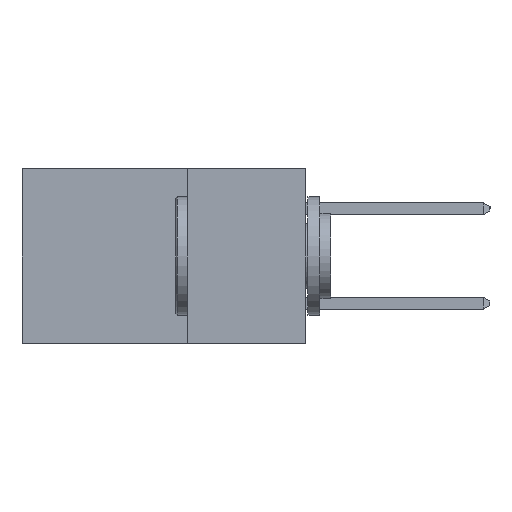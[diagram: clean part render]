
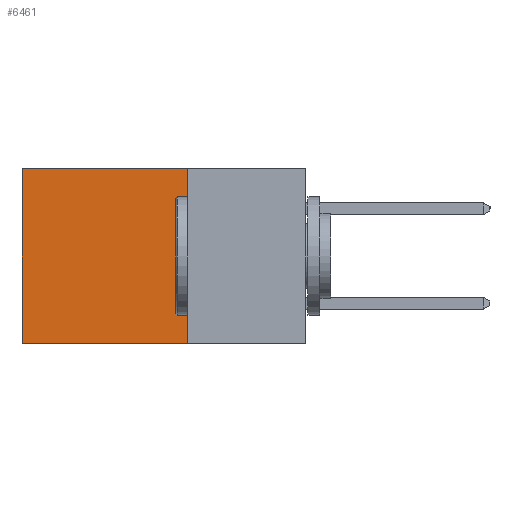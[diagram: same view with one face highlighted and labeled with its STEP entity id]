
A CAD part, left-side view. The second image highlights one B-rep face of the part: STEP entity #6461.
In plain terms, the highlighted planar face has unit normal (-1, 0, 0).
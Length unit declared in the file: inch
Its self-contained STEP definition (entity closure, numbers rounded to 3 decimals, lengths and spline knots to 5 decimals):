
#2274 = VECTOR ( 'NONE', #8849, 39.37008 ) ;
#3377 = EDGE_CURVE ( 'NONE', #10340, #13075, #22124, .T. ) ;
#3886 = VERTEX_POINT ( 'NONE', #10291 ) ;
#3919 = CARTESIAN_POINT ( 'NONE',  ( 0.2615, 0.25, 0. ) ) ;
#4617 = CARTESIAN_POINT ( 'NONE',  ( 0.2615, 0.25, -0.37 ) ) ;
#4715 = LINE ( 'NONE', #7134, #2274 ) ;
#5074 = CARTESIAN_POINT ( 'NONE',  ( 0.2615, 0.25, -0.37 ) ) ;
#6045 = CARTESIAN_POINT ( 'NONE',  ( 0.2615, 0.25, -0.37 ) ) ;
#6405 = ORIENTED_EDGE ( 'NONE', *, *, #15888, .F. ) ;
#6461 = ADVANCED_FACE ( 'NONE', ( #10420 ), #21023, .F. ) ;
#7134 = CARTESIAN_POINT ( 'NONE',  ( 0.2615, 0.6, -0.37 ) ) ;
#8092 = VERTEX_POINT ( 'NONE', #20190 ) ;
#8849 = DIRECTION ( 'NONE',  ( 0., 0., -1. ) ) ;
#9092 = DIRECTION ( 'NONE',  ( 0., 1., 0. ) ) ;
#9520 = VECTOR ( 'NONE', #9092, 39.37008 ) ;
#9632 = EDGE_CURVE ( 'NONE', #10340, #8092, #20566, .T. ) ;
#10031 = DIRECTION ( 'NONE',  ( 0., 0., -1. ) ) ;
#10291 = CARTESIAN_POINT ( 'NONE',  ( 0.2615, 0.6, -0.37 ) ) ;
#10340 = VERTEX_POINT ( 'NONE', #3919 ) ;
#10420 = FACE_OUTER_BOUND ( 'NONE', #11072, .T. ) ;
#11072 = EDGE_LOOP ( 'NONE', ( #22861, #6405, #26795, #20142 ) ) ;
#11405 = CARTESIAN_POINT ( 'NONE',  ( 0.2615, 0.25, 0. ) ) ;
#12316 = EDGE_CURVE ( 'NONE', #8092, #3886, #4715, .T. ) ;
#12444 = VECTOR ( 'NONE', #12496, 39.37008 ) ;
#12496 = DIRECTION ( 'NONE',  ( 0., 1., 0. ) ) ;
#13075 = VERTEX_POINT ( 'NONE', #4617 ) ;
#15888 = EDGE_CURVE ( 'NONE', #13075, #3886, #24966, .T. ) ;
#16730 = DIRECTION ( 'NONE',  ( 1., 0., 0. ) ) ;
#17155 = CARTESIAN_POINT ( 'NONE',  ( 0.2615, 0.25, -0.37 ) ) ;
#17691 = AXIS2_PLACEMENT_3D ( 'NONE', #17155, #16730, #27895 ) ;
#20142 = ORIENTED_EDGE ( 'NONE', *, *, #9632, .T. ) ;
#20190 = CARTESIAN_POINT ( 'NONE',  ( 0.2615, 0.6, 0. ) ) ;
#20566 = LINE ( 'NONE', #11405, #9520 ) ;
#21023 = PLANE ( 'NONE',  #17691 ) ;
#22124 = LINE ( 'NONE', #5074, #22824 ) ;
#22824 = VECTOR ( 'NONE', #10031, 39.37008 ) ;
#22861 = ORIENTED_EDGE ( 'NONE', *, *, #12316, .T. ) ;
#24966 = LINE ( 'NONE', #6045, #12444 ) ;
#26795 = ORIENTED_EDGE ( 'NONE', *, *, #3377, .F. ) ;
#27895 = DIRECTION ( 'NONE',  ( 0., 0., -1. ) ) ;
